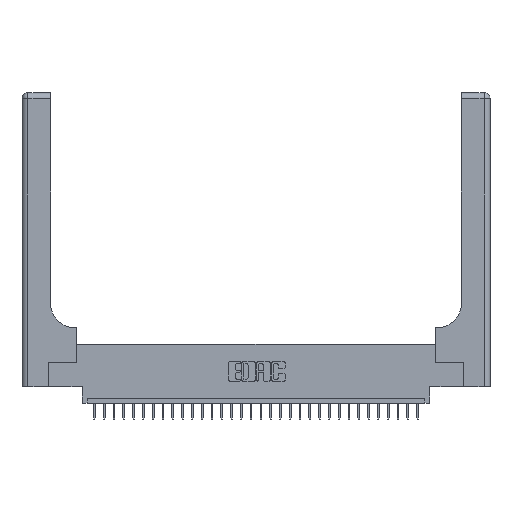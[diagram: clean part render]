
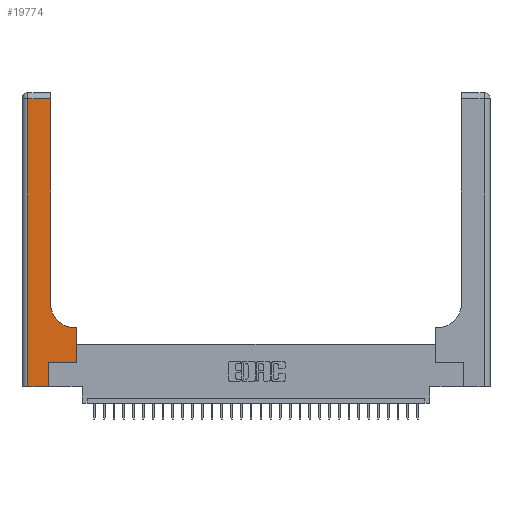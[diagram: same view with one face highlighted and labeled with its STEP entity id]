
A CAD part, top view. The second image highlights one B-rep face of the part: STEP entity #19774.
In plain terms, the highlighted planar face has unit normal (0, 0, 1).
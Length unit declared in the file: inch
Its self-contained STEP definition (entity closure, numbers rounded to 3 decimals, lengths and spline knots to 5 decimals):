
#459 = VECTOR ( 'NONE', #6877, 39.37008 ) ;
#667 = VECTOR ( 'NONE', #20407, 39.37008 ) ;
#697 = FACE_OUTER_BOUND ( 'NONE', #3492, .T. ) ;
#1442 = ORIENTED_EDGE ( 'NONE', *, *, #11856, .T. ) ;
#1530 = VERTEX_POINT ( 'NONE', #30013 ) ;
#2099 = LINE ( 'NONE', #12764, #16030 ) ;
#2150 = VERTEX_POINT ( 'NONE', #19979 ) ;
#2345 = DIRECTION ( 'NONE',  ( -1., 0., 0. ) ) ;
#2941 = EDGE_CURVE ( 'NONE', #27212, #2150, #16610, .T. ) ;
#2984 = LINE ( 'NONE', #15486, #667 ) ;
#3429 = VECTOR ( 'NONE', #5073, 39.37008 ) ;
#3484 = EDGE_CURVE ( 'NONE', #2150, #1530, #10749, .T. ) ;
#3492 = EDGE_LOOP ( 'NONE', ( #26195, #19286, #9544, #23188, #1442, #8286, #9406, #22338, #25020 ) ) ;
#3683 = AXIS2_PLACEMENT_3D ( 'NONE', #17155, #15113, #2345 ) ;
#3989 = EDGE_CURVE ( 'NONE', #6253, #4351, #2984, .T. ) ;
#4351 = VERTEX_POINT ( 'NONE', #26220 ) ;
#4670 = LINE ( 'NONE', #12149, #10049 ) ;
#5073 = DIRECTION ( 'NONE',  ( -1., 0., 0. ) ) ;
#5306 = DIRECTION ( 'NONE',  ( 0., 1., 0. ) ) ;
#5856 = EDGE_CURVE ( 'NONE', #6313, #11310, #2099, .T. ) ;
#6253 = VERTEX_POINT ( 'NONE', #11345 ) ;
#6275 = DIRECTION ( 'NONE',  ( 0., 0., -1. ) ) ;
#6313 = VERTEX_POINT ( 'NONE', #17502 ) ;
#6877 = DIRECTION ( 'NONE',  ( 1., 0., 0. ) ) ;
#7017 = LINE ( 'NONE', #14267, #459 ) ;
#7920 = VECTOR ( 'NONE', #14016, 39.37008 ) ;
#8059 = CIRCLE ( 'NONE', #19879, 0.25 ) ;
#8140 = EDGE_CURVE ( 'NONE', #17237, #20602, #7017, .T. ) ;
#8286 = ORIENTED_EDGE ( 'NONE', *, *, #5856, .T. ) ;
#8605 = CARTESIAN_POINT ( 'NONE',  ( 0.269, 0., 0.37 ) ) ;
#9406 = ORIENTED_EDGE ( 'NONE', *, *, #31794, .T. ) ;
#9544 = ORIENTED_EDGE ( 'NONE', *, *, #29265, .T. ) ;
#10049 = VECTOR ( 'NONE', #5306, 39.37008 ) ;
#10180 = CARTESIAN_POINT ( 'NONE',  ( 0., 2.94, 0.37 ) ) ;
#10749 = LINE ( 'NONE', #10180, #3429 ) ;
#11310 = VERTEX_POINT ( 'NONE', #20987 ) ;
#11326 = DIRECTION ( 'NONE',  ( 0., 1., 0. ) ) ;
#11345 = CARTESIAN_POINT ( 'NONE',  ( 0.5585, 0.6, 0.37 ) ) ;
#11856 = EDGE_CURVE ( 'NONE', #20602, #6313, #20502, .T. ) ;
#12149 = CARTESIAN_POINT ( 'NONE',  ( 0.5585, 0.25, 0.37 ) ) ;
#12764 = CARTESIAN_POINT ( 'NONE',  ( 0.269, 0.25, 0.37 ) ) ;
#14016 = DIRECTION ( 'NONE',  ( 0., -1., 0. ) ) ;
#14057 = EDGE_CURVE ( 'NONE', #4351, #27212, #8059, .T. ) ;
#14267 = CARTESIAN_POINT ( 'NONE',  ( 0., 0., 0.37 ) ) ;
#15078 = VECTOR ( 'NONE', #11326, 39.37008 ) ;
#15113 = DIRECTION ( 'NONE',  ( 0., 0., -1. ) ) ;
#15486 = CARTESIAN_POINT ( 'NONE',  ( 0.2915, 0.6, 0.37 ) ) ;
#15911 = VECTOR ( 'NONE', #26248, 39.37008 ) ;
#15937 = CARTESIAN_POINT ( 'NONE',  ( 0.06, 3., 0.37 ) ) ;
#16030 = VECTOR ( 'NONE', #30164, 39.37008 ) ;
#16610 = LINE ( 'NONE', #28547, #15078 ) ;
#17155 = CARTESIAN_POINT ( 'NONE',  ( 0., 3., 0.37 ) ) ;
#17237 = VERTEX_POINT ( 'NONE', #19319 ) ;
#17502 = CARTESIAN_POINT ( 'NONE',  ( 0.269, 0.25, 0.37 ) ) ;
#17566 = PLANE ( 'NONE',  #3683 ) ;
#18480 = DIRECTION ( 'NONE',  ( 1., 0., 0. ) ) ;
#19286 = ORIENTED_EDGE ( 'NONE', *, *, #3484, .T. ) ;
#19319 = CARTESIAN_POINT ( 'NONE',  ( 0.06, 0., 0.37 ) ) ;
#19774 = ADVANCED_FACE ( 'NONE', ( #697 ), #17566, .F. ) ;
#19879 = AXIS2_PLACEMENT_3D ( 'NONE', #20980, #6275, #18480 ) ;
#19979 = CARTESIAN_POINT ( 'NONE',  ( 0.2915, 2.94, 0.37 ) ) ;
#20407 = DIRECTION ( 'NONE',  ( -1., 0., 0. ) ) ;
#20502 = LINE ( 'NONE', #26031, #15911 ) ;
#20602 = VERTEX_POINT ( 'NONE', #8605 ) ;
#20980 = CARTESIAN_POINT ( 'NONE',  ( 0.5415, 0.85, 0.37 ) ) ;
#20987 = CARTESIAN_POINT ( 'NONE',  ( 0.5585, 0.25, 0.37 ) ) ;
#22338 = ORIENTED_EDGE ( 'NONE', *, *, #3989, .T. ) ;
#23188 = ORIENTED_EDGE ( 'NONE', *, *, #8140, .T. ) ;
#25020 = ORIENTED_EDGE ( 'NONE', *, *, #14057, .T. ) ;
#26031 = CARTESIAN_POINT ( 'NONE',  ( 0.269, 0., 0.37 ) ) ;
#26195 = ORIENTED_EDGE ( 'NONE', *, *, #2941, .T. ) ;
#26220 = CARTESIAN_POINT ( 'NONE',  ( 0.5415, 0.6, 0.37 ) ) ;
#26248 = DIRECTION ( 'NONE',  ( 0., 1., 0. ) ) ;
#27212 = VERTEX_POINT ( 'NONE', #30001 ) ;
#28547 = CARTESIAN_POINT ( 'NONE',  ( 0.2915, 3., 0.37 ) ) ;
#29265 = EDGE_CURVE ( 'NONE', #1530, #17237, #29595, .T. ) ;
#29595 = LINE ( 'NONE', #15937, #7920 ) ;
#30001 = CARTESIAN_POINT ( 'NONE',  ( 0.2915, 0.85, 0.37 ) ) ;
#30013 = CARTESIAN_POINT ( 'NONE',  ( 0.06, 2.94, 0.37 ) ) ;
#30164 = DIRECTION ( 'NONE',  ( 1., 0., 0. ) ) ;
#31794 = EDGE_CURVE ( 'NONE', #11310, #6253, #4670, .T. ) ;
